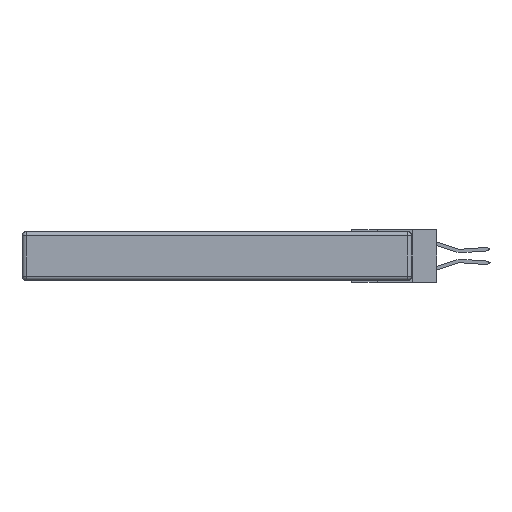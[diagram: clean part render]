
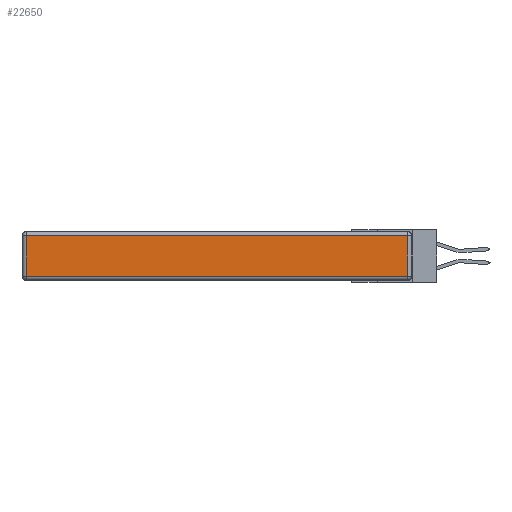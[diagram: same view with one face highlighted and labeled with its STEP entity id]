
A CAD part, left-side view. The second image highlights one B-rep face of the part: STEP entity #22650.
In plain terms, the highlighted planar face has unit normal (-1, 0, 0).
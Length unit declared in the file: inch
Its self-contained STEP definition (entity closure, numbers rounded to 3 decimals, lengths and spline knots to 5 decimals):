
#1555 = PLANE ( 'NONE',  #10161 ) ;
#3062 = CARTESIAN_POINT ( 'NONE',  ( 0., 0., -0.313 ) ) ;
#3366 = VECTOR ( 'NONE', #15697, 39.37008 ) ;
#3497 = ORIENTED_EDGE ( 'NONE', *, *, #26588, .T. ) ;
#4387 = LINE ( 'NONE', #18624, #12219 ) ;
#6659 = LINE ( 'NONE', #21131, #23696 ) ;
#7952 = ORIENTED_EDGE ( 'NONE', *, *, #24228, .T. ) ;
#8634 = DIRECTION ( 'NONE',  ( 0., 0., -1. ) ) ;
#8950 = LINE ( 'NONE', #13023, #3366 ) ;
#9982 = VERTEX_POINT ( 'NONE', #24395 ) ;
#10161 = AXIS2_PLACEMENT_3D ( 'NONE', #20359, #24839, #14279 ) ;
#12219 = VECTOR ( 'NONE', #24579, 39.37008 ) ;
#13023 = CARTESIAN_POINT ( 'NONE',  ( 0., 0.03, -0.343 ) ) ;
#13223 = CARTESIAN_POINT ( 'NONE',  ( 0., 2.72, -0.03 ) ) ;
#13452 = DIRECTION ( 'NONE',  ( 0., -1., 0. ) ) ;
#14279 = DIRECTION ( 'NONE',  ( 0., 0., 1. ) ) ;
#14405 = EDGE_CURVE ( 'NONE', #18772, #17383, #4387, .T. ) ;
#15007 = EDGE_CURVE ( 'NONE', #17383, #23352, #6659, .T. ) ;
#15197 = ORIENTED_EDGE ( 'NONE', *, *, #14405, .T. ) ;
#15697 = DIRECTION ( 'NONE',  ( 0., 0., 1. ) ) ;
#15855 = ORIENTED_EDGE ( 'NONE', *, *, #15007, .T. ) ;
#17222 = FACE_OUTER_BOUND ( 'NONE', #23710, .T. ) ;
#17383 = VERTEX_POINT ( 'NONE', #13223 ) ;
#18624 = CARTESIAN_POINT ( 'NONE',  ( 0., 2.75, -0.03 ) ) ;
#18772 = VERTEX_POINT ( 'NONE', #22805 ) ;
#20359 = CARTESIAN_POINT ( 'NONE',  ( 0., 0., -0.343 ) ) ;
#20599 = VECTOR ( 'NONE', #13452, 39.37008 ) ;
#21131 = CARTESIAN_POINT ( 'NONE',  ( 0., 2.72, -0.343 ) ) ;
#22554 = LINE ( 'NONE', #3062, #20599 ) ;
#22650 = ADVANCED_FACE ( 'NONE', ( #17222 ), #1555, .T. ) ;
#22805 = CARTESIAN_POINT ( 'NONE',  ( 0., 0.03, -0.03 ) ) ;
#23352 = VERTEX_POINT ( 'NONE', #25199 ) ;
#23696 = VECTOR ( 'NONE', #8634, 39.37008 ) ;
#23710 = EDGE_LOOP ( 'NONE', ( #3497, #7952, #15197, #15855 ) ) ;
#24228 = EDGE_CURVE ( 'NONE', #9982, #18772, #8950, .T. ) ;
#24395 = CARTESIAN_POINT ( 'NONE',  ( 0., 0.03, -0.313 ) ) ;
#24579 = DIRECTION ( 'NONE',  ( 0., 1., 0. ) ) ;
#24839 = DIRECTION ( 'NONE',  ( -1., 0., 0. ) ) ;
#25199 = CARTESIAN_POINT ( 'NONE',  ( 0., 2.72, -0.313 ) ) ;
#26588 = EDGE_CURVE ( 'NONE', #23352, #9982, #22554, .T. ) ;
